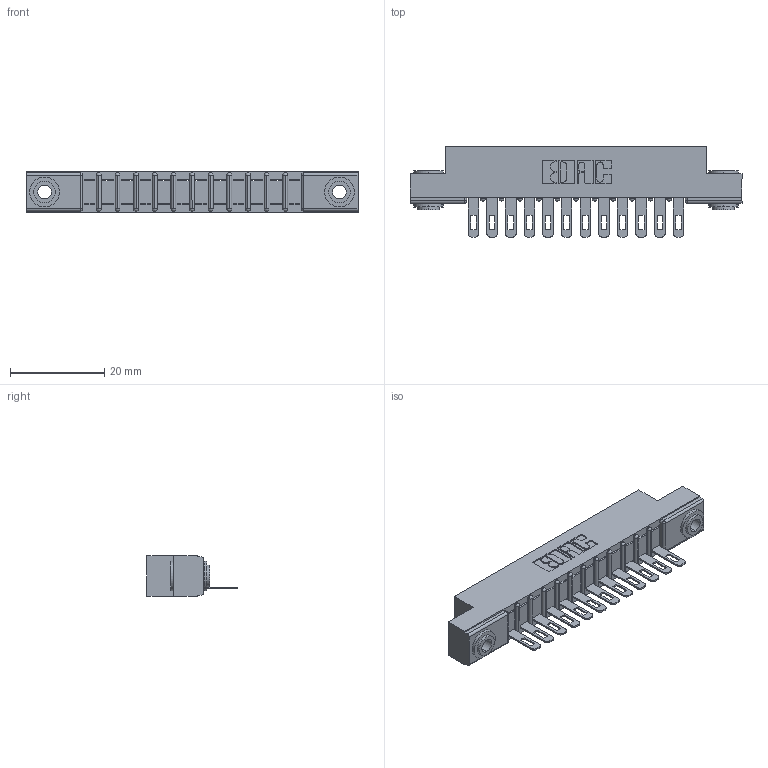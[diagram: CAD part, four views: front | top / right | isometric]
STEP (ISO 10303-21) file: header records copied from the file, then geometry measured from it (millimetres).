
FILE_DESCRIPTION (( 'STEP AP203' ), '1' );
FILE_NAME ('357-012-405-103.STEP', '2020-09-30T10:41:35', ( '' ), ( '' ), 'SwSTEP 2.0', 'SolidWorks 2020', '' );
FILE_SCHEMA (( 'CONFIG_CONTROL_DESIGN' ));
Length unit declared in the file: inch
Products named in the file (4): 357-012-405-103; 307-290-001_505; 307 Part_.156 Dia Mounting Holes; 345-250-002_345-250-002-102
Assembly tree (15 placements, depth 2):
  357-012-405-103
    307 Part_.156 Dia Mounting Holes
    307-290-001_505  x12
    345-250-002_345-250-002-102  x2
Bounding box: 70.56 x 19.18 x 8.71 mm (x, y, z)
Volume: 4497.4 mm3; surface area: 6946.2 mm2
Topology: 15 solids, 15 shells, 855 faces, 2379 edges, 1530 vertices
Faces by surface type: plane 526, cylinder 295, sphere 26, cone 8
Entity records: 15025 total; most frequent: CARTESIAN_POINT 2497, ORIENTED_EDGE 2474, DIRECTION 2463, EDGE_CURVE 1237, VECTOR 927, LINE 927, VERTEX_POINT 802, AXIS2_PLACEMENT_3D 768
